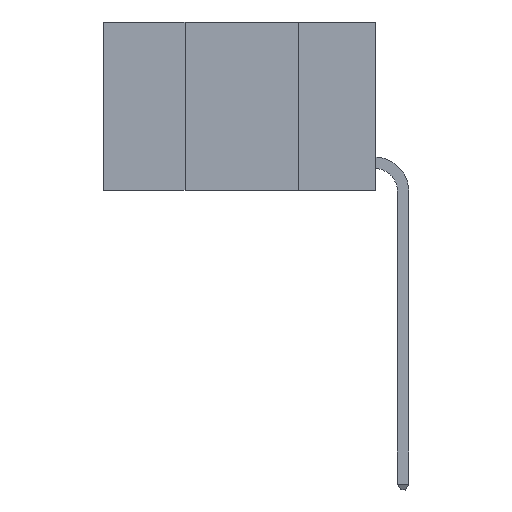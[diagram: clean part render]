
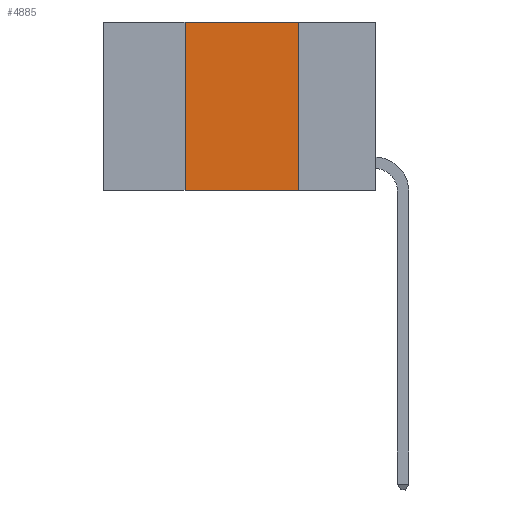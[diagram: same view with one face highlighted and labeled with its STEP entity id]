
A CAD part, left-side view. The second image highlights one B-rep face of the part: STEP entity #4885.
In plain terms, the highlighted planar face has unit normal (-1, 0, 0).
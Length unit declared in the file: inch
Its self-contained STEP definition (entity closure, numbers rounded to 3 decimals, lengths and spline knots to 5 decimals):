
#119 = CARTESIAN_POINT ( 'NONE',  ( 0., 0.17, 0. ) ) ;
#1195 = DIRECTION ( 'NONE',  ( 0., 0., -1. ) ) ;
#1274 = LINE ( 'NONE', #7299, #12379 ) ;
#1387 = CARTESIAN_POINT ( 'NONE',  ( 0., 0.17, 0. ) ) ;
#1931 = CARTESIAN_POINT ( 'NONE',  ( 0., 0.42, -0.37 ) ) ;
#2541 = CARTESIAN_POINT ( 'NONE',  ( 0., 0.6, 0. ) ) ;
#2826 = EDGE_CURVE ( 'NONE', #8054, #11039, #11899, .T. ) ;
#2827 = DIRECTION ( 'NONE',  ( 1., 0., 0. ) ) ;
#3308 = VECTOR ( 'NONE', #3622, 39.37008 ) ;
#3622 = DIRECTION ( 'NONE',  ( 0., -1., 0. ) ) ;
#4885 = ADVANCED_FACE ( 'NONE', ( #9450 ), #12453, .F. ) ;
#5502 = CARTESIAN_POINT ( 'NONE',  ( 0., 0.42, 0. ) ) ;
#5658 = AXIS2_PLACEMENT_3D ( 'NONE', #7126, #2827, #10387 ) ;
#6235 = DIRECTION ( 'NONE',  ( 0., -1., 0. ) ) ;
#6418 = EDGE_CURVE ( 'NONE', #13760, #10071, #1274, .T. ) ;
#6880 = CARTESIAN_POINT ( 'NONE',  ( 0., 0.42, 0. ) ) ;
#7126 = CARTESIAN_POINT ( 'NONE',  ( 0., 0.6, 0. ) ) ;
#7299 = CARTESIAN_POINT ( 'NONE',  ( 0., 0.6, -0.37 ) ) ;
#7945 = DIRECTION ( 'NONE',  ( 0., 0., 1. ) ) ;
#7999 = ORIENTED_EDGE ( 'NONE', *, *, #11605, .F. ) ;
#8054 = VERTEX_POINT ( 'NONE', #5502 ) ;
#9172 = VECTOR ( 'NONE', #7945, 39.37008 ) ;
#9450 = FACE_OUTER_BOUND ( 'NONE', #12302, .T. ) ;
#9855 = LINE ( 'NONE', #6880, #9172 ) ;
#10071 = VERTEX_POINT ( 'NONE', #11200 ) ;
#10387 = DIRECTION ( 'NONE',  ( 0., 0., -1. ) ) ;
#10534 = ORIENTED_EDGE ( 'NONE', *, *, #12748, .F. ) ;
#10857 = ORIENTED_EDGE ( 'NONE', *, *, #6418, .T. ) ;
#11039 = VERTEX_POINT ( 'NONE', #1387 ) ;
#11160 = LINE ( 'NONE', #119, #13595 ) ;
#11200 = CARTESIAN_POINT ( 'NONE',  ( 0., 0.17, -0.37 ) ) ;
#11605 = EDGE_CURVE ( 'NONE', #13760, #8054, #9855, .T. ) ;
#11899 = LINE ( 'NONE', #2541, #3308 ) ;
#12302 = EDGE_LOOP ( 'NONE', ( #10534, #13310, #7999, #10857 ) ) ;
#12379 = VECTOR ( 'NONE', #6235, 39.37008 ) ;
#12453 = PLANE ( 'NONE',  #5658 ) ;
#12748 = EDGE_CURVE ( 'NONE', #11039, #10071, #11160, .T. ) ;
#13310 = ORIENTED_EDGE ( 'NONE', *, *, #2826, .F. ) ;
#13595 = VECTOR ( 'NONE', #1195, 39.37008 ) ;
#13760 = VERTEX_POINT ( 'NONE', #1931 ) ;
